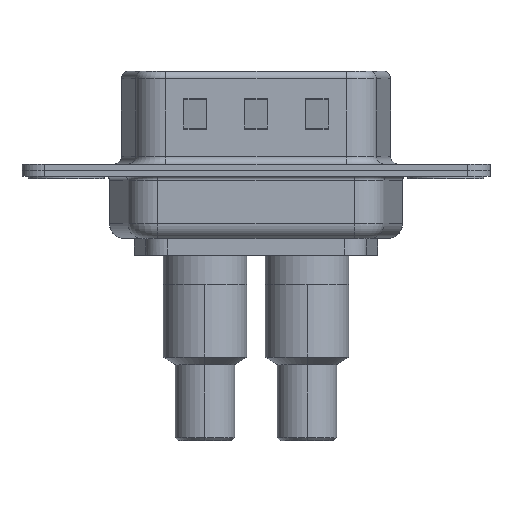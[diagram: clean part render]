
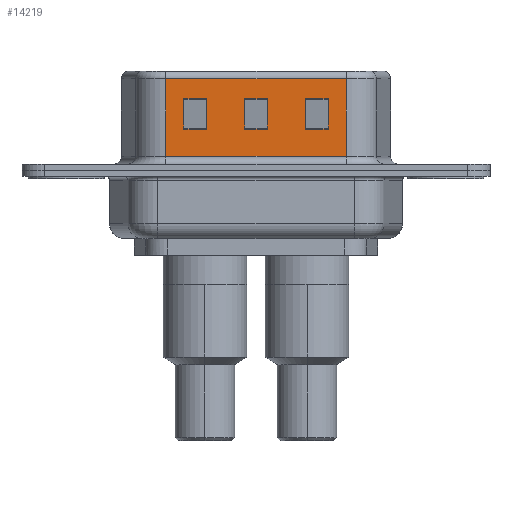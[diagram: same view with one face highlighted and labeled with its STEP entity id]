
A CAD part, front view. The second image highlights one B-rep face of the part: STEP entity #14219.
In plain terms, the highlighted planar face has unit normal (0, -1, 0).
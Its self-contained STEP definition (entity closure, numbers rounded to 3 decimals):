
#288 = LINE ( 'NONE', #9344, #10927 ) ;
#333 = EDGE_CURVE ( 'NONE', #10606, #6470, #9889, .T. ) ;
#366 = EDGE_LOOP ( 'NONE', ( #8031, #12030, #17008, #8708 ) ) ;
#514 = FACE_BOUND ( 'NONE', #2809, .T. ) ;
#622 = DIRECTION ( 'NONE',  ( 0., 0., 1. ) ) ;
#647 = CARTESIAN_POINT ( 'NONE',  ( 11.75, -4.58, 2.705 ) ) ;
#863 = EDGE_CURVE ( 'NONE', #12002, #3973, #16075, .T. ) ;
#989 = EDGE_CURVE ( 'NONE', #8685, #5405, #288, .T. ) ;
#1049 = VECTOR ( 'NONE', #2529, 1000. ) ;
#1071 = VECTOR ( 'NONE', #3490, 1000. ) ;
#1129 = ORIENTED_EDGE ( 'NONE', *, *, #989, .T. ) ;
#1216 = CARTESIAN_POINT ( 'NONE',  ( 18.45, -4.58, 6.02 ) ) ;
#1347 = DIRECTION ( 'NONE',  ( 0., 0., -1. ) ) ;
#1484 = CARTESIAN_POINT ( 'NONE',  ( 13.25, -4.58, 4.705 ) ) ;
#1597 = EDGE_LOOP ( 'NONE', ( #7181, #13450, #10384, #8699 ) ) ;
#1669 = EDGE_CURVE ( 'NONE', #6481, #6461, #1746, .T. ) ;
#1746 = LINE ( 'NONE', #8456, #15416 ) ;
#1802 = CARTESIAN_POINT ( 'NONE',  ( 18.45, -4.58, 6.02 ) ) ;
#1838 = DIRECTION ( 'NONE',  ( -1., 0., 0. ) ) ;
#2006 = VERTEX_POINT ( 'NONE', #1802 ) ;
#2023 = DIRECTION ( 'NONE',  ( -1., 0., 0. ) ) ;
#2258 = EDGE_CURVE ( 'NONE', #6461, #8685, #4886, .T. ) ;
#2270 = VECTOR ( 'NONE', #8084, 1000. ) ;
#2529 = DIRECTION ( 'NONE',  ( 0., 0., -1. ) ) ;
#2588 = CARTESIAN_POINT ( 'NONE',  ( 18.45, -4.58, 6.52 ) ) ;
#2809 = EDGE_LOOP ( 'NONE', ( #11322, #8551, #6382, #1129 ) ) ;
#2922 = EDGE_CURVE ( 'NONE', #5405, #6481, #4642, .T. ) ;
#3031 = DIRECTION ( 'NONE',  ( 1., 0., 0. ) ) ;
#3211 = DIRECTION ( 'NONE',  ( 0., 0., -1. ) ) ;
#3333 = CARTESIAN_POINT ( 'NONE',  ( 7.75, -4.58, 4.705 ) ) ;
#3438 = CARTESIAN_POINT ( 'NONE',  ( 7.75, -4.58, 2.705 ) ) ;
#3464 = EDGE_CURVE ( 'NONE', #2006, #8329, #4208, .T. ) ;
#3486 = CARTESIAN_POINT ( 'NONE',  ( 13.25, -4.58, 2.705 ) ) ;
#3490 = DIRECTION ( 'NONE',  ( 1., 0., 0. ) ) ;
#3619 = EDGE_CURVE ( 'NONE', #6470, #8092, #13122, .T. ) ;
#3728 = EDGE_CURVE ( 'NONE', #16630, #10606, #7460, .T. ) ;
#3884 = LINE ( 'NONE', #6968, #7350 ) ;
#3973 = VERTEX_POINT ( 'NONE', #16715 ) ;
#4089 = VERTEX_POINT ( 'NONE', #15407 ) ;
#4114 = FACE_BOUND ( 'NONE', #366, .T. ) ;
#4208 = LINE ( 'NONE', #2588, #1049 ) ;
#4318 = CARTESIAN_POINT ( 'NONE',  ( 9.25, -4.58, 6.52 ) ) ;
#4642 = LINE ( 'NONE', #15840, #1071 ) ;
#4764 = DIRECTION ( 'NONE',  ( 0., 0., -1. ) ) ;
#4886 = LINE ( 'NONE', #6031, #8343 ) ;
#4959 = EDGE_CURVE ( 'NONE', #8092, #16630, #6245, .T. ) ;
#5163 = LINE ( 'NONE', #11021, #11794 ) ;
#5190 = VECTOR ( 'NONE', #4764, 1000. ) ;
#5259 = CARTESIAN_POINT ( 'NONE',  ( 18.45, -4.58, 0.9 ) ) ;
#5405 = VERTEX_POINT ( 'NONE', #8135 ) ;
#5687 = VERTEX_POINT ( 'NONE', #14058 ) ;
#5888 = AXIS2_PLACEMENT_3D ( 'NONE', #8122, #16123, #8180 ) ;
#6031 = CARTESIAN_POINT ( 'NONE',  ( 18.45, -4.58, 2.705 ) ) ;
#6056 = EDGE_CURVE ( 'NONE', #2006, #5687, #15058, .T. ) ;
#6245 = LINE ( 'NONE', #4318, #12460 ) ;
#6382 = ORIENTED_EDGE ( 'NONE', *, *, #2258, .T. ) ;
#6386 = VECTOR ( 'NONE', #11568, 1000. ) ;
#6461 = VERTEX_POINT ( 'NONE', #3486 ) ;
#6470 = VERTEX_POINT ( 'NONE', #3333 ) ;
#6481 = VERTEX_POINT ( 'NONE', #1484 ) ;
#6613 = LINE ( 'NONE', #10800, #2270 ) ;
#6737 = VECTOR ( 'NONE', #10920, 1000. ) ;
#6782 = EDGE_CURVE ( 'NONE', #3973, #14753, #5163, .T. ) ;
#6905 = ORIENTED_EDGE ( 'NONE', *, *, #6782, .T. ) ;
#6968 = CARTESIAN_POINT ( 'NONE',  ( 18.45, -4.58, 0.9 ) ) ;
#7126 = LINE ( 'NONE', #9578, #6737 ) ;
#7181 = ORIENTED_EDGE ( 'NONE', *, *, #3464, .F. ) ;
#7338 = EDGE_CURVE ( 'NONE', #9888, #8329, #3884, .T. ) ;
#7350 = VECTOR ( 'NONE', #3031, 1000. ) ;
#7460 = LINE ( 'NONE', #14369, #7888 ) ;
#7888 = VECTOR ( 'NONE', #1838, 1000. ) ;
#7988 = CARTESIAN_POINT ( 'NONE',  ( 17.25, -4.58, 4.705 ) ) ;
#7996 = FACE_BOUND ( 'NONE', #14481, .T. ) ;
#8031 = ORIENTED_EDGE ( 'NONE', *, *, #4959, .T. ) ;
#8084 = DIRECTION ( 'NONE',  ( -1., 0., 0. ) ) ;
#8092 = VERTEX_POINT ( 'NONE', #11286 ) ;
#8122 = CARTESIAN_POINT ( 'NONE',  ( 18.45, -4.58, 6.52 ) ) ;
#8135 = CARTESIAN_POINT ( 'NONE',  ( 11.75, -4.58, 4.705 ) ) ;
#8180 = DIRECTION ( 'NONE',  ( 0., 0., 1. ) ) ;
#8264 = DIRECTION ( 'NONE',  ( 1., 0., 0. ) ) ;
#8329 = VERTEX_POINT ( 'NONE', #5259 ) ;
#8343 = VECTOR ( 'NONE', #15246, 1000. ) ;
#8456 = CARTESIAN_POINT ( 'NONE',  ( 13.25, -4.58, 6.52 ) ) ;
#8551 = ORIENTED_EDGE ( 'NONE', *, *, #1669, .T. ) ;
#8685 = VERTEX_POINT ( 'NONE', #647 ) ;
#8699 = ORIENTED_EDGE ( 'NONE', *, *, #7338, .T. ) ;
#8708 = ORIENTED_EDGE ( 'NONE', *, *, #3619, .T. ) ;
#8724 = VECTOR ( 'NONE', #8264, 1000. ) ;
#9344 = CARTESIAN_POINT ( 'NONE',  ( 11.75, -4.58, 6.52 ) ) ;
#9578 = CARTESIAN_POINT ( 'NONE',  ( 6.55, -4.58, 6.52 ) ) ;
#9888 = VERTEX_POINT ( 'NONE', #13626 ) ;
#9889 = LINE ( 'NONE', #15264, #6386 ) ;
#10384 = ORIENTED_EDGE ( 'NONE', *, *, #15313, .T. ) ;
#10606 = VERTEX_POINT ( 'NONE', #3438 ) ;
#10800 = CARTESIAN_POINT ( 'NONE',  ( 22.45, -4.58, 2.705 ) ) ;
#10822 = CARTESIAN_POINT ( 'NONE',  ( 9.25, -4.58, 2.705 ) ) ;
#10920 = DIRECTION ( 'NONE',  ( 0., 0., -1. ) ) ;
#10927 = VECTOR ( 'NONE', #622, 1000. ) ;
#11021 = CARTESIAN_POINT ( 'NONE',  ( 22.45, -4.58, 4.705 ) ) ;
#11078 = DIRECTION ( 'NONE',  ( 1., 0., 0. ) ) ;
#11113 = CARTESIAN_POINT ( 'NONE',  ( 15.75, -4.58, 6.52 ) ) ;
#11286 = CARTESIAN_POINT ( 'NONE',  ( 9.25, -4.58, 4.705 ) ) ;
#11322 = ORIENTED_EDGE ( 'NONE', *, *, #2922, .T. ) ;
#11441 = ORIENTED_EDGE ( 'NONE', *, *, #863, .T. ) ;
#11568 = DIRECTION ( 'NONE',  ( 0., 0., 1. ) ) ;
#11613 = VECTOR ( 'NONE', #2023, 1000. ) ;
#11794 = VECTOR ( 'NONE', #11078, 1000. ) ;
#11890 = ORIENTED_EDGE ( 'NONE', *, *, #13061, .T. ) ;
#12002 = VERTEX_POINT ( 'NONE', #14759 ) ;
#12030 = ORIENTED_EDGE ( 'NONE', *, *, #3728, .T. ) ;
#12460 = VECTOR ( 'NONE', #1347, 1000. ) ;
#12584 = VECTOR ( 'NONE', #15340, 1000. ) ;
#13061 = EDGE_CURVE ( 'NONE', #4089, #12002, #6613, .T. ) ;
#13122 = LINE ( 'NONE', #13619, #8724 ) ;
#13377 = EDGE_CURVE ( 'NONE', #14753, #4089, #15701, .T. ) ;
#13450 = ORIENTED_EDGE ( 'NONE', *, *, #6056, .T. ) ;
#13482 = PLANE ( 'NONE',  #5888 ) ;
#13516 = ORIENTED_EDGE ( 'NONE', *, *, #13377, .T. ) ;
#13619 = CARTESIAN_POINT ( 'NONE',  ( 14.45, -4.58, 4.705 ) ) ;
#13626 = CARTESIAN_POINT ( 'NONE',  ( 6.55, -4.58, 0.9 ) ) ;
#14058 = CARTESIAN_POINT ( 'NONE',  ( 6.55, -4.58, 6.02 ) ) ;
#14219 = ADVANCED_FACE ( 'NONE', ( #4114, #7996, #514, #14232 ), #13482, .F. ) ;
#14232 = FACE_OUTER_BOUND ( 'NONE', #1597, .T. ) ;
#14369 = CARTESIAN_POINT ( 'NONE',  ( 14.45, -4.58, 2.705 ) ) ;
#14481 = EDGE_LOOP ( 'NONE', ( #13516, #11890, #11441, #6905 ) ) ;
#14753 = VERTEX_POINT ( 'NONE', #7988 ) ;
#14759 = CARTESIAN_POINT ( 'NONE',  ( 15.75, -4.58, 2.705 ) ) ;
#15058 = LINE ( 'NONE', #1216, #11613 ) ;
#15246 = DIRECTION ( 'NONE',  ( -1., 0., 0. ) ) ;
#15264 = CARTESIAN_POINT ( 'NONE',  ( 7.75, -4.58, 6.52 ) ) ;
#15313 = EDGE_CURVE ( 'NONE', #5687, #9888, #7126, .T. ) ;
#15340 = DIRECTION ( 'NONE',  ( 0., 0., 1. ) ) ;
#15407 = CARTESIAN_POINT ( 'NONE',  ( 17.25, -4.58, 2.705 ) ) ;
#15416 = VECTOR ( 'NONE', #3211, 1000. ) ;
#15701 = LINE ( 'NONE', #16650, #5190 ) ;
#15840 = CARTESIAN_POINT ( 'NONE',  ( 18.45, -4.58, 4.705 ) ) ;
#16075 = LINE ( 'NONE', #11113, #12584 ) ;
#16123 = DIRECTION ( 'NONE',  ( 0., 1., 0. ) ) ;
#16630 = VERTEX_POINT ( 'NONE', #10822 ) ;
#16650 = CARTESIAN_POINT ( 'NONE',  ( 17.25, -4.58, 6.52 ) ) ;
#16715 = CARTESIAN_POINT ( 'NONE',  ( 15.75, -4.58, 4.705 ) ) ;
#17008 = ORIENTED_EDGE ( 'NONE', *, *, #333, .T. ) ;
